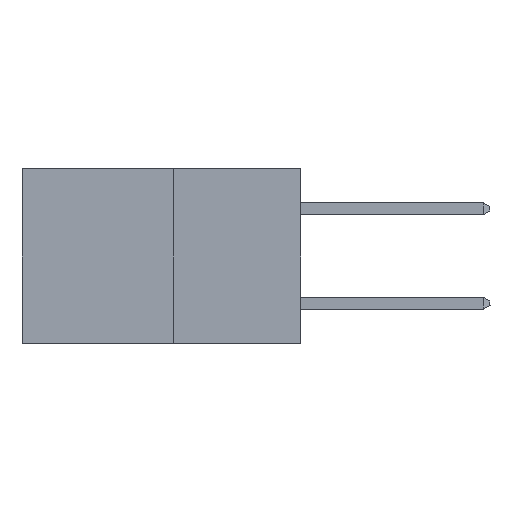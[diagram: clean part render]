
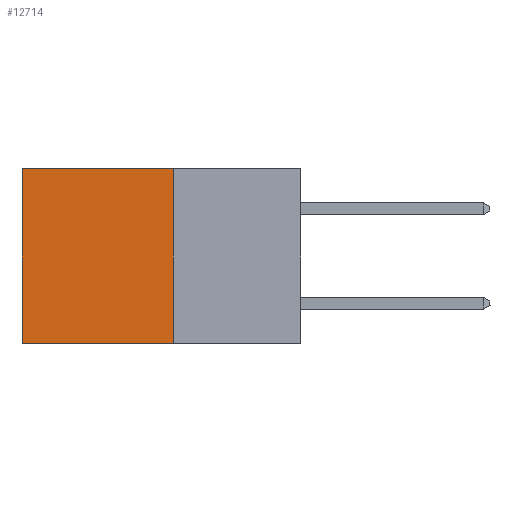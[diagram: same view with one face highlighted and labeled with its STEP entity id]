
A CAD part, left-side view. The second image highlights one B-rep face of the part: STEP entity #12714.
In plain terms, the highlighted planar face has unit normal (-1, 0, 0).
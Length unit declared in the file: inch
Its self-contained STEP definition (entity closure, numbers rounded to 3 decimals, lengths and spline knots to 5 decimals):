
#930 = DIRECTION ( 'NONE',  ( 0., 1., 0. ) ) ;
#1126 = LINE ( 'NONE', #12077, #5647 ) ;
#3033 = AXIS2_PLACEMENT_3D ( 'NONE', #5346, #20718, #9227 ) ;
#3991 = EDGE_CURVE ( 'NONE', #19974, #11442, #11080, .T. ) ;
#4844 = ORIENTED_EDGE ( 'NONE', *, *, #17533, .F. ) ;
#5346 = CARTESIAN_POINT ( 'NONE',  ( 0.277, 0.27, -0.37 ) ) ;
#5647 = VECTOR ( 'NONE', #14004, 39.37008 ) ;
#7167 = EDGE_LOOP ( 'NONE', ( #8828, #4844, #9949, #14353 ) ) ;
#8274 = CARTESIAN_POINT ( 'NONE',  ( 0.277, 0.27, -0.37 ) ) ;
#8436 = VERTEX_POINT ( 'NONE', #17444 ) ;
#8828 = ORIENTED_EDGE ( 'NONE', *, *, #13063, .T. ) ;
#8987 = FACE_OUTER_BOUND ( 'NONE', #7167, .T. ) ;
#9227 = DIRECTION ( 'NONE',  ( 0., 0., -1. ) ) ;
#9560 = LINE ( 'NONE', #14166, #19189 ) ;
#9949 = ORIENTED_EDGE ( 'NONE', *, *, #13134, .F. ) ;
#10522 = CARTESIAN_POINT ( 'NONE',  ( 0.277, 0.27, 0. ) ) ;
#10524 = CARTESIAN_POINT ( 'NONE',  ( 0.277, 0.27, -0.37 ) ) ;
#11080 = LINE ( 'NONE', #10522, #11677 ) ;
#11442 = VERTEX_POINT ( 'NONE', #21017 ) ;
#11604 = VECTOR ( 'NONE', #15894, 39.37008 ) ;
#11677 = VECTOR ( 'NONE', #930, 39.37008 ) ;
#12077 = CARTESIAN_POINT ( 'NONE',  ( 0.277, 0.59, -0.37 ) ) ;
#12714 = ADVANCED_FACE ( 'NONE', ( #8987 ), #24496, .F. ) ;
#13063 = EDGE_CURVE ( 'NONE', #11442, #8436, #1126, .T. ) ;
#13134 = EDGE_CURVE ( 'NONE', #19974, #17650, #9560, .T. ) ;
#14004 = DIRECTION ( 'NONE',  ( 0., 0., -1. ) ) ;
#14166 = CARTESIAN_POINT ( 'NONE',  ( 0.277, 0.27, -0.37 ) ) ;
#14353 = ORIENTED_EDGE ( 'NONE', *, *, #3991, .T. ) ;
#14783 = CARTESIAN_POINT ( 'NONE',  ( 0.277, 0.27, 0. ) ) ;
#15894 = DIRECTION ( 'NONE',  ( 0., 1., 0. ) ) ;
#16108 = DIRECTION ( 'NONE',  ( 0., 0., -1. ) ) ;
#16122 = LINE ( 'NONE', #8274, #11604 ) ;
#17444 = CARTESIAN_POINT ( 'NONE',  ( 0.277, 0.59, -0.37 ) ) ;
#17533 = EDGE_CURVE ( 'NONE', #17650, #8436, #16122, .T. ) ;
#17650 = VERTEX_POINT ( 'NONE', #10524 ) ;
#19189 = VECTOR ( 'NONE', #16108, 39.37008 ) ;
#19974 = VERTEX_POINT ( 'NONE', #14783 ) ;
#20718 = DIRECTION ( 'NONE',  ( 1., 0., 0. ) ) ;
#21017 = CARTESIAN_POINT ( 'NONE',  ( 0.277, 0.59, 0. ) ) ;
#24496 = PLANE ( 'NONE',  #3033 ) ;
